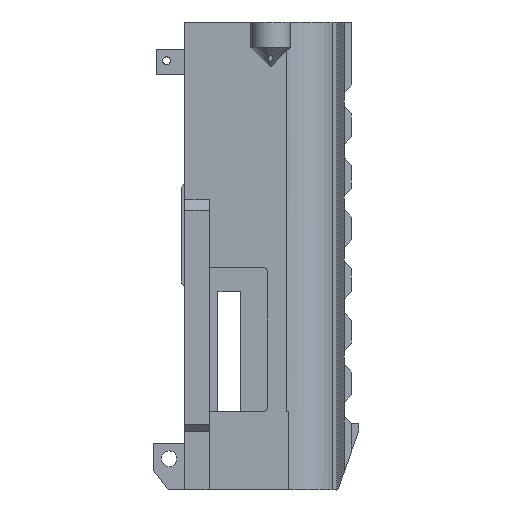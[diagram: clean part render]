
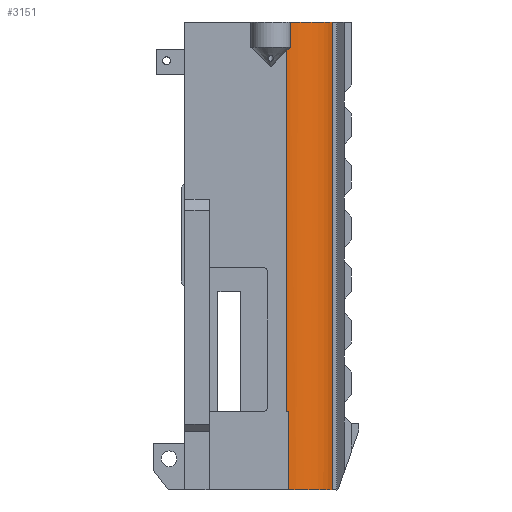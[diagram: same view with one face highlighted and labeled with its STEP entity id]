
A CAD part, left-side view. The second image highlights one B-rep face of the part: STEP entity #3151.
In plain terms, the highlighted cylindrical face has radius 20.1 mm (diameter 40.2 mm), a partial arc.
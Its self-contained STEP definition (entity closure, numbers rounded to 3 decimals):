
#50 = CARTESIAN_POINT ( 'NONE',  ( -19.05, 47.913, 0. ) ) ;
#280 = VERTEX_POINT ( 'NONE', #6244 ) ;
#382 = LINE ( 'NONE', #5103, #7860 ) ;
#532 = CYLINDRICAL_SURFACE ( 'NONE', #671, 20.1 ) ;
#671 = AXIS2_PLACEMENT_3D ( 'NONE', #50, #6641, #7347 ) ;
#694 = DIRECTION ( 'NONE',  ( -1., 0., 0. ) ) ;
#710 = CARTESIAN_POINT ( 'NONE',  ( -19.05, 48.472, 20.092 ) ) ;
#880 = AXIS2_PLACEMENT_3D ( 'NONE', #7281, #694, #2927 ) ;
#1073 = AXIS2_PLACEMENT_3D ( 'NONE', #3912, #4734, #6113 ) ;
#1138 = VERTEX_POINT ( 'NONE', #2994 ) ;
#1310 = FACE_OUTER_BOUND ( 'NONE', #5091, .T. ) ;
#1433 = ORIENTED_EDGE ( 'NONE', *, *, #7207, .T. ) ;
#1611 = EDGE_CURVE ( 'NONE', #5540, #2224, #5753, .T. ) ;
#1937 = AXIS2_PLACEMENT_3D ( 'NONE', #3852, #8872, #6737 ) ;
#2115 = CARTESIAN_POINT ( 'NONE',  ( -167.482, 49.3, 20.052 ) ) ;
#2172 = CARTESIAN_POINT ( 'NONE',  ( -166.095, 47.913, 20.1 ) ) ;
#2224 = VERTEX_POINT ( 'NONE', #3703 ) ;
#2318 = CARTESIAN_POINT ( 'NONE',  ( -19.05, 49.3, 20.052 ) ) ;
#2570 = CARTESIAN_POINT ( 'NONE',  ( -19.05, 47.913, 20.1 ) ) ;
#2927 = DIRECTION ( 'NONE',  ( 0., -1., 0. ) ) ;
#2935 = DIRECTION ( 'NONE',  ( 1., 0., 0. ) ) ;
#2954 = EDGE_CURVE ( 'NONE', #280, #1138, #8824, .T. ) ;
#2994 = CARTESIAN_POINT ( 'NONE',  ( -166.095, 47.913, 20.1 ) ) ;
#3151 = ADVANCED_FACE ( 'NONE', ( #1310 ), #532, .T. ) ;
#3166 = ORIENTED_EDGE ( 'NONE', *, *, #5243, .T. ) ;
#3180 = EDGE_CURVE ( 'NONE', #8340, #5257, #4357, .T. ) ;
#3335 = ORIENTED_EDGE ( 'NONE', *, *, #5758, .F. ) ;
#3359 = VERTEX_POINT ( 'NONE', #3369 ) ;
#3369 = CARTESIAN_POINT ( 'NONE',  ( -19.05, 47.913, 20.1 ) ) ;
#3703 = CARTESIAN_POINT ( 'NONE',  ( 12.7, 66.303, 8.113 ) ) ;
#3852 = CARTESIAN_POINT ( 'NONE',  ( -177.682, 47.913, 0. ) ) ;
#3912 = CARTESIAN_POINT ( 'NONE',  ( 12.7, 47.913, 0. ) ) ;
#4209 = VECTOR ( 'NONE', #6050, 1000. ) ;
#4321 = CARTESIAN_POINT ( 'NONE',  ( 12.7, 48.472, 20.092 ) ) ;
#4357 = CIRCLE ( 'NONE', #1937, 20.1 ) ;
#4488 = EDGE_CURVE ( 'NONE', #6547, #5540, #382, .T. ) ;
#4734 = DIRECTION ( 'NONE',  ( -1., 0., 0. ) ) ;
#4738 = CIRCLE ( 'NONE', #880, 20.1 ) ;
#5091 = EDGE_LOOP ( 'NONE', ( #3166, #5687, #1433, #8950, #3335, #6654, #6938, #6718 ) ) ;
#5103 = CARTESIAN_POINT ( 'NONE',  ( -194.05, 48.472, 20.092 ) ) ;
#5243 = EDGE_CURVE ( 'NONE', #2224, #8340, #9240, .T. ) ;
#5257 = VERTEX_POINT ( 'NONE', #6790 ) ;
#5389 = VECTOR ( 'NONE', #5985, 1000. ) ;
#5540 = VERTEX_POINT ( 'NONE', #4321 ) ;
#5687 = ORIENTED_EDGE ( 'NONE', *, *, #3180, .T. ) ;
#5753 = CIRCLE ( 'NONE', #1073, 20.1 ) ;
#5758 = EDGE_CURVE ( 'NONE', #3359, #1138, #8004, .T. ) ;
#5985 = DIRECTION ( 'NONE',  ( -1., 0., 0. ) ) ;
#6050 = DIRECTION ( 'NONE',  ( 1., 0., 0. ) ) ;
#6113 = DIRECTION ( 'NONE',  ( 0., -1., 0. ) ) ;
#6244 = CARTESIAN_POINT ( 'NONE',  ( -167.482, 49.3, 20.052 ) ) ;
#6525 = VECTOR ( 'NONE', #9124, 1000. ) ;
#6547 = VERTEX_POINT ( 'NONE', #710 ) ;
#6606 = LINE ( 'NONE', #2318, #4209 ) ;
#6641 = DIRECTION ( 'NONE',  ( 1., 0., 0. ) ) ;
#6654 = ORIENTED_EDGE ( 'NONE', *, *, #8459, .T. ) ;
#6718 = ORIENTED_EDGE ( 'NONE', *, *, #1611, .T. ) ;
#6737 = DIRECTION ( 'NONE',  ( 0., -1., 0. ) ) ;
#6790 = CARTESIAN_POINT ( 'NONE',  ( -177.682, 49.3, 20.052 ) ) ;
#6938 = ORIENTED_EDGE ( 'NONE', *, *, #4488, .T. ) ;
#7207 = EDGE_CURVE ( 'NONE', #5257, #280, #6606, .T. ) ;
#7231 = CARTESIAN_POINT ( 'NONE',  ( -166.554, 48.372, 20.1 ) ) ;
#7281 = CARTESIAN_POINT ( 'NONE',  ( -19.05, 47.913, 0. ) ) ;
#7347 = DIRECTION ( 'NONE',  ( 0., -1., 0. ) ) ;
#7399 = CARTESIAN_POINT ( 'NONE',  ( -19.05, 66.303, 8.113 ) ) ;
#7860 = VECTOR ( 'NONE', #2935, 1000. ) ;
#8004 = LINE ( 'NONE', #2570, #6525 ) ;
#8340 = VERTEX_POINT ( 'NONE', #8534 ) ;
#8459 = EDGE_CURVE ( 'NONE', #3359, #6547, #4738, .T. ) ;
#8534 = CARTESIAN_POINT ( 'NONE',  ( -177.682, 66.303, 8.113 ) ) ;
#8824 = B_SPLINE_CURVE_WITH_KNOTS ( 'NONE', 3,
 ( #2115, #9279, #7231, #2172 ),
 .UNSPECIFIED., .F., .F.,
 ( 4, 4 ),
 ( -5.303, -5.108 ),
 .UNSPECIFIED. ) ;
#8872 = DIRECTION ( 'NONE',  ( 1., 0., 0. ) ) ;
#8950 = ORIENTED_EDGE ( 'NONE', *, *, #2954, .T. ) ;
#9124 = DIRECTION ( 'NONE',  ( -1., 0., 0. ) ) ;
#9240 = LINE ( 'NONE', #7399, #5389 ) ;
#9279 = CARTESIAN_POINT ( 'NONE',  ( -167.017, 48.835, 20.084 ) ) ;
